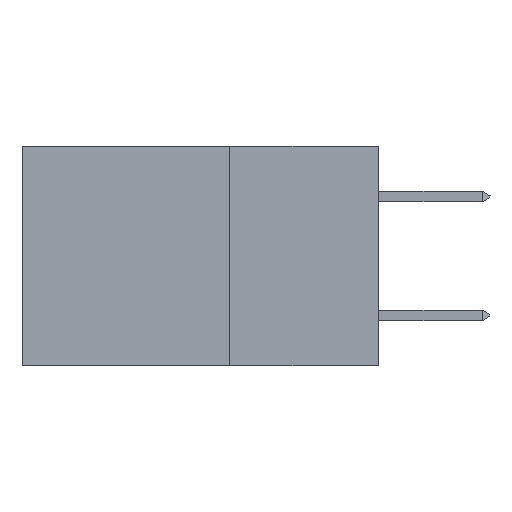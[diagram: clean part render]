
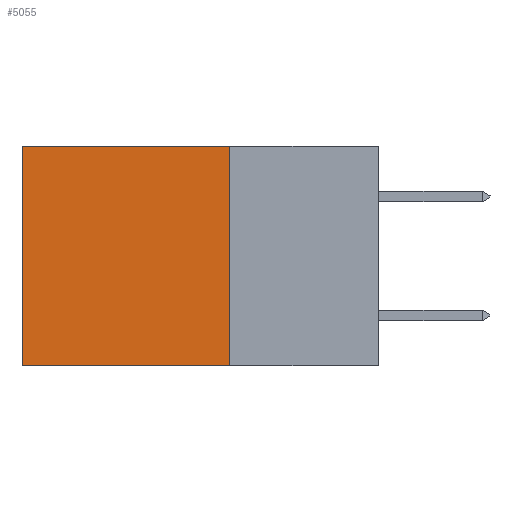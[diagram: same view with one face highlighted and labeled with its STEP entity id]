
A CAD part, left-side view. The second image highlights one B-rep face of the part: STEP entity #5055.
In plain terms, the highlighted planar face has unit normal (-1, 0, 0).
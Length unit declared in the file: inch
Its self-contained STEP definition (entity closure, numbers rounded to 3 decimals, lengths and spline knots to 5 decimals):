
#266 = VECTOR ( 'NONE', #5811, 39.37008 ) ;
#334 = VERTEX_POINT ( 'NONE', #9386 ) ;
#860 = VERTEX_POINT ( 'NONE', #8364 ) ;
#1364 = CARTESIAN_POINT ( 'NONE',  ( 0.2615, 0.25, -0.37 ) ) ;
#1541 = FACE_OUTER_BOUND ( 'NONE', #9202, .T. ) ;
#1585 = ORIENTED_EDGE ( 'NONE', *, *, #8170, .T. ) ;
#1626 = CARTESIAN_POINT ( 'NONE',  ( 0.2615, 0.25, -0.37 ) ) ;
#1794 = LINE ( 'NONE', #1626, #6243 ) ;
#2066 = EDGE_CURVE ( 'NONE', #4731, #11359, #10159, .T. ) ;
#2374 = LINE ( 'NONE', #6130, #5174 ) ;
#3463 = EDGE_CURVE ( 'NONE', #4731, #860, #1794, .T. ) ;
#4731 = VERTEX_POINT ( 'NONE', #5468 ) ;
#5055 = ADVANCED_FACE ( 'NONE', ( #1541 ), #5993, .F. ) ;
#5174 = VECTOR ( 'NONE', #7890, 39.37008 ) ;
#5468 = CARTESIAN_POINT ( 'NONE',  ( 0.2615, 0.25, 0. ) ) ;
#5508 = AXIS2_PLACEMENT_3D ( 'NONE', #1364, #8780, #7702 ) ;
#5811 = DIRECTION ( 'NONE',  ( 0., 1., 0. ) ) ;
#5993 = PLANE ( 'NONE',  #5508 ) ;
#6011 = VECTOR ( 'NONE', #10939, 39.37008 ) ;
#6130 = CARTESIAN_POINT ( 'NONE',  ( 0.2615, 0.6, -0.37 ) ) ;
#6243 = VECTOR ( 'NONE', #8871, 39.37008 ) ;
#7286 = CARTESIAN_POINT ( 'NONE',  ( 0.2615, 0.6, 0. ) ) ;
#7698 = CARTESIAN_POINT ( 'NONE',  ( 0.2615, 0.25, -0.37 ) ) ;
#7702 = DIRECTION ( 'NONE',  ( 0., 0., -1. ) ) ;
#7890 = DIRECTION ( 'NONE',  ( 0., 0., -1. ) ) ;
#8075 = ORIENTED_EDGE ( 'NONE', *, *, #11024, .F. ) ;
#8170 = EDGE_CURVE ( 'NONE', #11359, #334, #2374, .T. ) ;
#8364 = CARTESIAN_POINT ( 'NONE',  ( 0.2615, 0.25, -0.37 ) ) ;
#8434 = ORIENTED_EDGE ( 'NONE', *, *, #3463, .F. ) ;
#8598 = LINE ( 'NONE', #7698, #266 ) ;
#8780 = DIRECTION ( 'NONE',  ( 1., 0., 0. ) ) ;
#8871 = DIRECTION ( 'NONE',  ( 0., 0., -1. ) ) ;
#8964 = CARTESIAN_POINT ( 'NONE',  ( 0.2615, 0.25, 0. ) ) ;
#9148 = ORIENTED_EDGE ( 'NONE', *, *, #2066, .T. ) ;
#9202 = EDGE_LOOP ( 'NONE', ( #1585, #8075, #8434, #9148 ) ) ;
#9386 = CARTESIAN_POINT ( 'NONE',  ( 0.2615, 0.6, -0.37 ) ) ;
#10159 = LINE ( 'NONE', #8964, #6011 ) ;
#10939 = DIRECTION ( 'NONE',  ( 0., 1., 0. ) ) ;
#11024 = EDGE_CURVE ( 'NONE', #860, #334, #8598, .T. ) ;
#11359 = VERTEX_POINT ( 'NONE', #7286 ) ;
